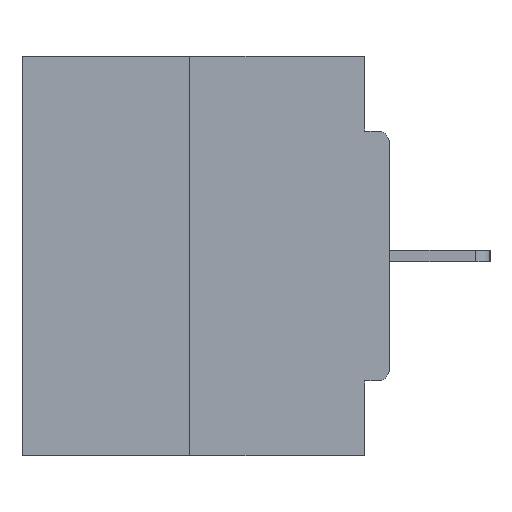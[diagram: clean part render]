
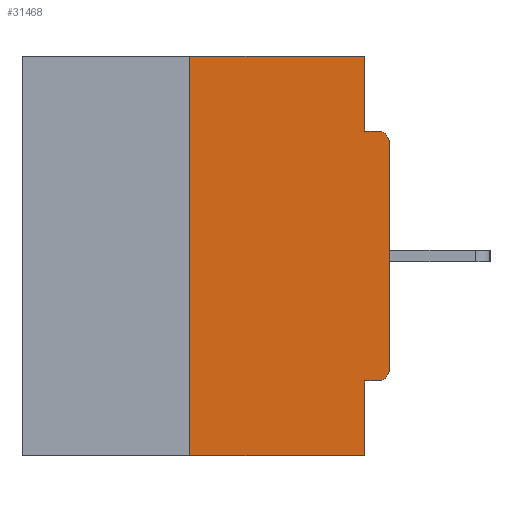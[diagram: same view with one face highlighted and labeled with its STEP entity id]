
A CAD part, left-side view. The second image highlights one B-rep face of the part: STEP entity #31468.
In plain terms, the highlighted planar face has unit normal (-1, 0, 0).
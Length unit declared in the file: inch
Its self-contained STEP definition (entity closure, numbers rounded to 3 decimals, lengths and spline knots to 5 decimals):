
#125 = CARTESIAN_POINT ( 'NONE',  ( 0., 0.031, -0.5 ) ) ;
#889 = EDGE_CURVE ( 'NONE', #11604, #8514, #10870, .T. ) ;
#1116 = CARTESIAN_POINT ( 'NONE',  ( 0., 0.031, 0. ) ) ;
#1649 = VECTOR ( 'NONE', #31146, 39.37008 ) ;
#2180 = EDGE_CURVE ( 'NONE', #17383, #29838, #11371, .T. ) ;
#2476 = ORIENTED_EDGE ( 'NONE', *, *, #2180, .F. ) ;
#2930 = EDGE_CURVE ( 'NONE', #22987, #19880, #4219, .T. ) ;
#3308 = ORIENTED_EDGE ( 'NONE', *, *, #889, .F. ) ;
#3649 = ORIENTED_EDGE ( 'NONE', *, *, #28906, .F. ) ;
#4030 = DIRECTION ( 'NONE',  ( 1., 0., 0. ) ) ;
#4157 = ORIENTED_EDGE ( 'NONE', *, *, #10113, .F. ) ;
#4158 = CIRCLE ( 'NONE', #28228, 0.015 ) ;
#4219 = CIRCLE ( 'NONE', #28290, 0.015 ) ;
#4896 = VECTOR ( 'NONE', #9982, 39.37008 ) ;
#5297 = ORIENTED_EDGE ( 'NONE', *, *, #10613, .T. ) ;
#5799 = LINE ( 'NONE', #31562, #7004 ) ;
#6973 = CARTESIAN_POINT ( 'NONE',  ( 0., 0.25, -0.5 ) ) ;
#7004 = VECTOR ( 'NONE', #28739, 39.37008 ) ;
#7245 = AXIS2_PLACEMENT_3D ( 'NONE', #26994, #4030, #21612 ) ;
#7893 = CARTESIAN_POINT ( 'NONE',  ( 0., 0.25, 0. ) ) ;
#8343 = DIRECTION ( 'NONE',  ( 0., 0., -1. ) ) ;
#8504 = EDGE_CURVE ( 'NONE', #8862, #29939, #4158, .T. ) ;
#8514 = VERTEX_POINT ( 'NONE', #1116 ) ;
#8846 = CARTESIAN_POINT ( 'NONE',  ( 0., 0.015, -0.1085 ) ) ;
#8862 = VERTEX_POINT ( 'NONE', #28221 ) ;
#9970 = CARTESIAN_POINT ( 'NONE',  ( 0., 0.015, -0.3915 ) ) ;
#9982 = DIRECTION ( 'NONE',  ( 0., -1., 0. ) ) ;
#10113 = EDGE_CURVE ( 'NONE', #22987, #17383, #5799, .T. ) ;
#10219 = CARTESIAN_POINT ( 'NONE',  ( 0., 0., 0. ) ) ;
#10289 = VECTOR ( 'NONE', #16746, 39.37008 ) ;
#10319 = EDGE_CURVE ( 'NONE', #19880, #8862, #10566, .T. ) ;
#10566 = LINE ( 'NONE', #10219, #1649 ) ;
#10601 = CARTESIAN_POINT ( 'NONE',  ( 0., 0., -0.3915 ) ) ;
#10613 = EDGE_CURVE ( 'NONE', #16664, #29838, #22366, .T. ) ;
#10870 = LINE ( 'NONE', #31463, #27168 ) ;
#11371 = LINE ( 'NONE', #16244, #24723 ) ;
#11415 = VECTOR ( 'NONE', #13931, 39.37008 ) ;
#11604 = VERTEX_POINT ( 'NONE', #7893 ) ;
#11749 = VERTEX_POINT ( 'NONE', #29659 ) ;
#13361 = ORIENTED_EDGE ( 'NONE', *, *, #8504, .T. ) ;
#13931 = DIRECTION ( 'NONE',  ( 0., 0., -1. ) ) ;
#13989 = ORIENTED_EDGE ( 'NONE', *, *, #10319, .T. ) ;
#14260 = ORIENTED_EDGE ( 'NONE', *, *, #16102, .F. ) ;
#16102 = EDGE_CURVE ( 'NONE', #11749, #29939, #17229, .T. ) ;
#16244 = CARTESIAN_POINT ( 'NONE',  ( 0., 0.031, -0.5 ) ) ;
#16312 = CARTESIAN_POINT ( 'NONE',  ( 0., 0.031, -0.4065 ) ) ;
#16448 = CARTESIAN_POINT ( 'NONE',  ( 0., 0.031, 0. ) ) ;
#16664 = VERTEX_POINT ( 'NONE', #6973 ) ;
#16746 = DIRECTION ( 'NONE',  ( 0., -1., 0. ) ) ;
#16857 = LINE ( 'NONE', #27083, #17784 ) ;
#17229 = LINE ( 'NONE', #32126, #10289 ) ;
#17383 = VERTEX_POINT ( 'NONE', #16312 ) ;
#17784 = VECTOR ( 'NONE', #31932, 39.37008 ) ;
#17969 = ORIENTED_EDGE ( 'NONE', *, *, #27972, .F. ) ;
#19211 = DIRECTION ( 'NONE',  ( -1., 0., 0. ) ) ;
#19880 = VERTEX_POINT ( 'NONE', #10601 ) ;
#21612 = DIRECTION ( 'NONE',  ( 0., 0., -1. ) ) ;
#21745 = DIRECTION ( 'NONE',  ( 0., 0., -1. ) ) ;
#22366 = LINE ( 'NONE', #32910, #4896 ) ;
#22987 = VERTEX_POINT ( 'NONE', #31076 ) ;
#23071 = CARTESIAN_POINT ( 'NONE',  ( 0., 0.015, -0.0935 ) ) ;
#23739 = ORIENTED_EDGE ( 'NONE', *, *, #2930, .T. ) ;
#23919 = EDGE_LOOP ( 'NONE', ( #3308, #3649, #5297, #2476, #4157, #23739, #13989, #13361, #14260, #17969 ) ) ;
#24624 = PLANE ( 'NONE',  #7245 ) ;
#24723 = VECTOR ( 'NONE', #21745, 39.37008 ) ;
#26335 = LINE ( 'NONE', #16448, #11415 ) ;
#26994 = CARTESIAN_POINT ( 'NONE',  ( 0., 0.46, 0. ) ) ;
#27083 = CARTESIAN_POINT ( 'NONE',  ( 0., 0.25, 0. ) ) ;
#27168 = VECTOR ( 'NONE', #31959, 39.37008 ) ;
#27972 = EDGE_CURVE ( 'NONE', #8514, #11749, #26335, .T. ) ;
#28218 = DIRECTION ( 'NONE',  ( 0., 0., -1. ) ) ;
#28221 = CARTESIAN_POINT ( 'NONE',  ( 0., 0., -0.1085 ) ) ;
#28228 = AXIS2_PLACEMENT_3D ( 'NONE', #8846, #19211, #8343 ) ;
#28290 = AXIS2_PLACEMENT_3D ( 'NONE', #9970, #30728, #28218 ) ;
#28739 = DIRECTION ( 'NONE',  ( 0., 1., 0. ) ) ;
#28906 = EDGE_CURVE ( 'NONE', #16664, #11604, #16857, .T. ) ;
#29659 = CARTESIAN_POINT ( 'NONE',  ( 0., 0.031, -0.0935 ) ) ;
#29838 = VERTEX_POINT ( 'NONE', #125 ) ;
#29939 = VERTEX_POINT ( 'NONE', #23071 ) ;
#30728 = DIRECTION ( 'NONE',  ( -1., 0., 0. ) ) ;
#31076 = CARTESIAN_POINT ( 'NONE',  ( 0., 0.015, -0.4065 ) ) ;
#31146 = DIRECTION ( 'NONE',  ( 0., 0., 1. ) ) ;
#31463 = CARTESIAN_POINT ( 'NONE',  ( 0., 0.46, 0. ) ) ;
#31468 = ADVANCED_FACE ( 'NONE', ( #32324 ), #24624, .F. ) ;
#31562 = CARTESIAN_POINT ( 'NONE',  ( 0., 0., -0.4065 ) ) ;
#31932 = DIRECTION ( 'NONE',  ( 0., 0., 1. ) ) ;
#31959 = DIRECTION ( 'NONE',  ( 0., -1., 0. ) ) ;
#32126 = CARTESIAN_POINT ( 'NONE',  ( 0., 0., -0.0935 ) ) ;
#32324 = FACE_OUTER_BOUND ( 'NONE', #23919, .T. ) ;
#32910 = CARTESIAN_POINT ( 'NONE',  ( 0., 0.46, -0.5 ) ) ;
